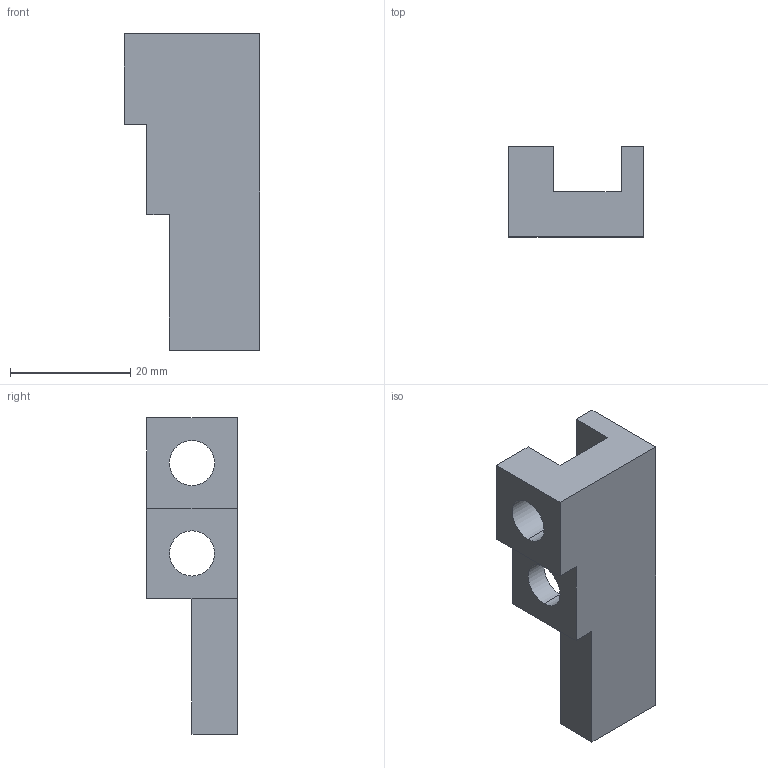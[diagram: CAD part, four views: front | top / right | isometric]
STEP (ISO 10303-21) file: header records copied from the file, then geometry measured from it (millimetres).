
FILE_DESCRIPTION (( 'STEP AP203' ), '1' );
FILE_NAME ('Bottom_Cover_Left.STEP', '2013-09-22T12:23:24', ( '' ), ( '' ), 'SwSTEP 2.0', 'SolidWorks 2013', '' );
FILE_SCHEMA (( 'CONFIG_CONTROL_DESIGN' ));
Length unit declared in the file: millimetre
Products named in the file (1): Bottom_Cover_Left
Bounding box: 22.5 x 15 x 52.5 mm (x, y, z)
Volume: 7955.9 mm3; surface area: 4379.3 mm2
Topology: 1 solids, 1 shells, 23 faces, 66 edges, 41 vertices
Faces by surface type: plane 17, cylinder 6
Entity records: 833 total; most frequent: ORIENTED_EDGE 132, CARTESIAN_POINT 131, DIRECTION 126, EDGE_CURVE 66, LINE 54, VECTOR 54, VERTEX_POINT 41, AXIS2_PLACEMENT_3D 36
